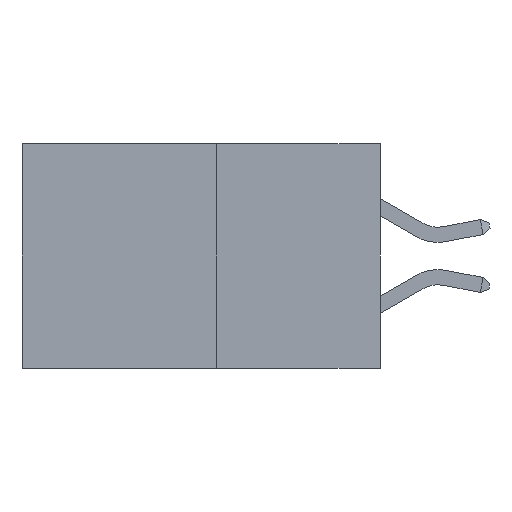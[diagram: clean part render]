
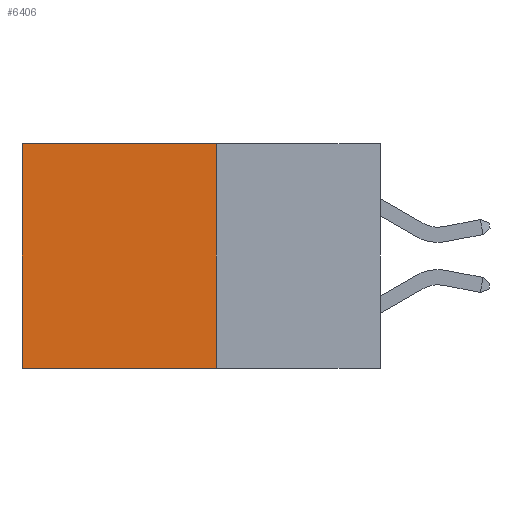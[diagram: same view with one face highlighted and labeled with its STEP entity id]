
A CAD part, left-side view. The second image highlights one B-rep face of the part: STEP entity #6406.
In plain terms, the highlighted planar face has unit normal (-1, 0, 0).
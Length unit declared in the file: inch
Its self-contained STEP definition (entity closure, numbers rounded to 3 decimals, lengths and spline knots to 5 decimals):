
#351 = DIRECTION ( 'NONE',  ( 0., 1., 0. ) ) ;
#375 = LINE ( 'NONE', #5580, #1929 ) ;
#535 = FACE_OUTER_BOUND ( 'NONE', #3803, .T. ) ;
#571 = ORIENTED_EDGE ( 'NONE', *, *, #2142, .F. ) ;
#658 = DIRECTION ( 'NONE',  ( 0., 0., -1. ) ) ;
#695 = VECTOR ( 'NONE', #5134, 39.37008 ) ;
#1217 = VECTOR ( 'NONE', #5896, 39.37008 ) ;
#1359 = VERTEX_POINT ( 'NONE', #2331 ) ;
#1797 = ORIENTED_EDGE ( 'NONE', *, *, #4893, .T. ) ;
#1929 = VECTOR ( 'NONE', #351, 39.37008 ) ;
#2009 = CARTESIAN_POINT ( 'NONE',  ( 0.277, 0.27, -0.37 ) ) ;
#2040 = CARTESIAN_POINT ( 'NONE',  ( 0.277, 0.27, 0. ) ) ;
#2045 = CARTESIAN_POINT ( 'NONE',  ( 0.277, 0.59, -0.37 ) ) ;
#2142 = EDGE_CURVE ( 'NONE', #6618, #3246, #5427, .T. ) ;
#2267 = ORIENTED_EDGE ( 'NONE', *, *, #3101, .F. ) ;
#2331 = CARTESIAN_POINT ( 'NONE',  ( 0.277, 0.59, 0. ) ) ;
#2488 = VECTOR ( 'NONE', #4826, 39.37008 ) ;
#2737 = LINE ( 'NONE', #2040, #1217 ) ;
#2819 = VERTEX_POINT ( 'NONE', #2045 ) ;
#3101 = EDGE_CURVE ( 'NONE', #3246, #2819, #375, .T. ) ;
#3170 = ORIENTED_EDGE ( 'NONE', *, *, #3464, .T. ) ;
#3246 = VERTEX_POINT ( 'NONE', #6628 ) ;
#3249 = PLANE ( 'NONE',  #7462 ) ;
#3464 = EDGE_CURVE ( 'NONE', #6618, #1359, #2737, .T. ) ;
#3803 = EDGE_LOOP ( 'NONE', ( #1797, #2267, #571, #3170 ) ) ;
#4529 = DIRECTION ( 'NONE',  ( 1., 0., 0. ) ) ;
#4734 = CARTESIAN_POINT ( 'NONE',  ( 0.277, 0.59, -0.37 ) ) ;
#4826 = DIRECTION ( 'NONE',  ( 0., 0., -1. ) ) ;
#4893 = EDGE_CURVE ( 'NONE', #1359, #2819, #7131, .T. ) ;
#5134 = DIRECTION ( 'NONE',  ( 0., 0., -1. ) ) ;
#5358 = CARTESIAN_POINT ( 'NONE',  ( 0.277, 0.27, 0. ) ) ;
#5427 = LINE ( 'NONE', #2009, #695 ) ;
#5580 = CARTESIAN_POINT ( 'NONE',  ( 0.277, 0.27, -0.37 ) ) ;
#5896 = DIRECTION ( 'NONE',  ( 0., 1., 0. ) ) ;
#6406 = ADVANCED_FACE ( 'NONE', ( #535 ), #3249, .F. ) ;
#6618 = VERTEX_POINT ( 'NONE', #5358 ) ;
#6628 = CARTESIAN_POINT ( 'NONE',  ( 0.277, 0.27, -0.37 ) ) ;
#7131 = LINE ( 'NONE', #4734, #2488 ) ;
#7462 = AXIS2_PLACEMENT_3D ( 'NONE', #7880, #4529, #658 ) ;
#7880 = CARTESIAN_POINT ( 'NONE',  ( 0.277, 0.27, -0.37 ) ) ;
